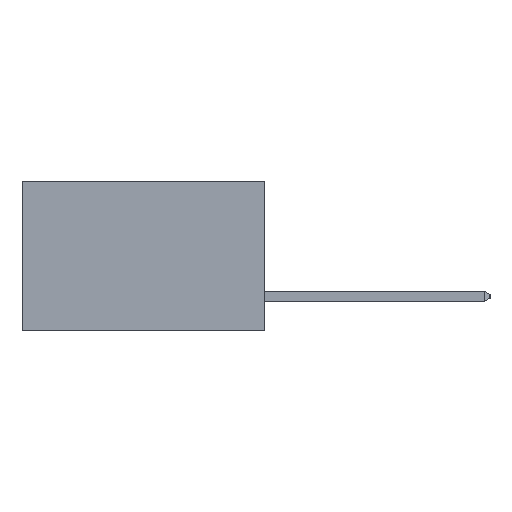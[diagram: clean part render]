
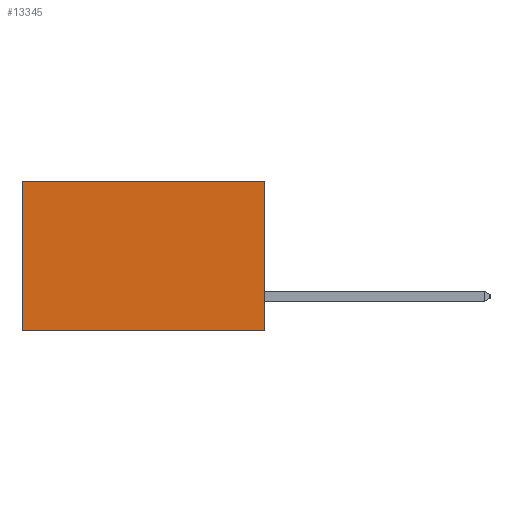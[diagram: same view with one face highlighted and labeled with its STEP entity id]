
A CAD part, left-side view. The second image highlights one B-rep face of the part: STEP entity #13345.
In plain terms, the highlighted planar face has unit normal (-1, 0, 0).
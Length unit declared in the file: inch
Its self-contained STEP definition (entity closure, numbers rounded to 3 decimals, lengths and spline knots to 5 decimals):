
#342 = EDGE_CURVE ( 'NONE', #9592, #8578, #7778, .T. ) ;
#611 = EDGE_CURVE ( 'NONE', #3898, #12621, #4767, .T. ) ;
#1666 = VECTOR ( 'NONE', #4245, 39.37008 ) ;
#1868 = CARTESIAN_POINT ( 'NONE',  ( 0.2615, 0.6, 0. ) ) ;
#2464 = ORIENTED_EDGE ( 'NONE', *, *, #342, .T. ) ;
#2935 = CARTESIAN_POINT ( 'NONE',  ( 0.2615, 0., 0. ) ) ;
#3256 = CARTESIAN_POINT ( 'NONE',  ( 0.2615, 0.6, -0.37 ) ) ;
#3693 = CARTESIAN_POINT ( 'NONE',  ( 0.2615, 0.6, -0.37 ) ) ;
#3898 = VERTEX_POINT ( 'NONE', #2935 ) ;
#4058 = AXIS2_PLACEMENT_3D ( 'NONE', #13970, #7050, #15087 ) ;
#4245 = DIRECTION ( 'NONE',  ( 0., 0., -1. ) ) ;
#4767 = LINE ( 'NONE', #6786, #13371 ) ;
#5017 = CARTESIAN_POINT ( 'NONE',  ( 0.2615, 0., -0.37 ) ) ;
#5144 = EDGE_CURVE ( 'NONE', #12621, #8578, #14058, .T. ) ;
#5462 = FACE_OUTER_BOUND ( 'NONE', #12873, .T. ) ;
#5734 = EDGE_CURVE ( 'NONE', #3898, #9592, #14556, .T. ) ;
#6057 = DIRECTION ( 'NONE',  ( 0., 1., 0. ) ) ;
#6786 = CARTESIAN_POINT ( 'NONE',  ( 0.2615, 0., -0.37 ) ) ;
#7050 = DIRECTION ( 'NONE',  ( 1., 0., 0. ) ) ;
#7778 = LINE ( 'NONE', #3256, #1666 ) ;
#8578 = VERTEX_POINT ( 'NONE', #3693 ) ;
#9201 = CARTESIAN_POINT ( 'NONE',  ( 0.2615, 0., -0.37 ) ) ;
#9592 = VERTEX_POINT ( 'NONE', #1868 ) ;
#9722 = DIRECTION ( 'NONE',  ( 0., 1., 0. ) ) ;
#9956 = CARTESIAN_POINT ( 'NONE',  ( 0.2615, 0., 0. ) ) ;
#10661 = VECTOR ( 'NONE', #6057, 39.37008 ) ;
#12476 = ORIENTED_EDGE ( 'NONE', *, *, #5144, .F. ) ;
#12621 = VERTEX_POINT ( 'NONE', #9201 ) ;
#12642 = ORIENTED_EDGE ( 'NONE', *, *, #5734, .T. ) ;
#12833 = PLANE ( 'NONE',  #4058 ) ;
#12873 = EDGE_LOOP ( 'NONE', ( #2464, #12476, #14069, #12642 ) ) ;
#13345 = ADVANCED_FACE ( 'NONE', ( #5462 ), #12833, .F. ) ;
#13371 = VECTOR ( 'NONE', #15270, 39.37008 ) ;
#13970 = CARTESIAN_POINT ( 'NONE',  ( 0.2615, 0., -0.37 ) ) ;
#14058 = LINE ( 'NONE', #5017, #10661 ) ;
#14069 = ORIENTED_EDGE ( 'NONE', *, *, #611, .F. ) ;
#14556 = LINE ( 'NONE', #9956, #14918 ) ;
#14918 = VECTOR ( 'NONE', #9722, 39.37008 ) ;
#15087 = DIRECTION ( 'NONE',  ( 0., 0., -1. ) ) ;
#15270 = DIRECTION ( 'NONE',  ( 0., 0., -1. ) ) ;
